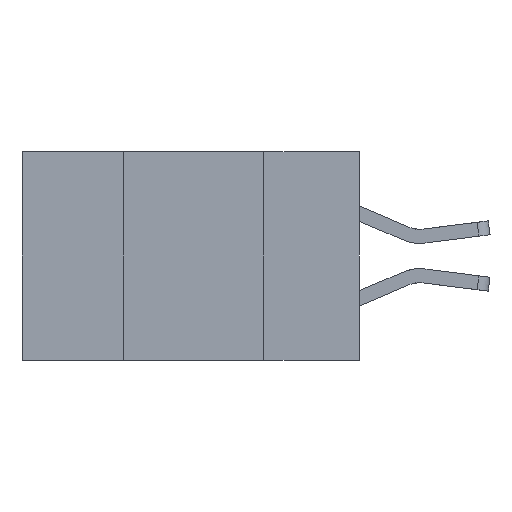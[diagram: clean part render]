
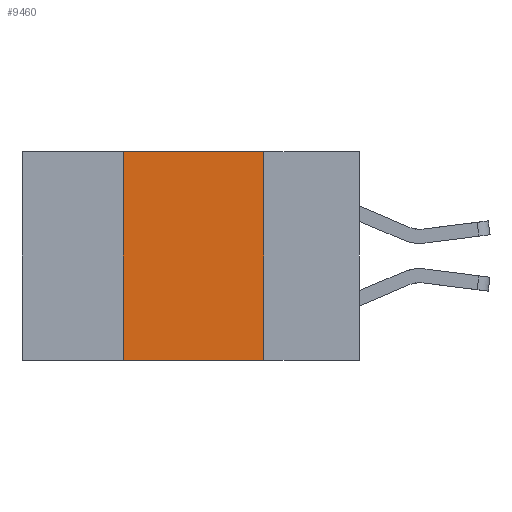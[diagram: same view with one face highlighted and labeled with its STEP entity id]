
A CAD part, left-side view. The second image highlights one B-rep face of the part: STEP entity #9460.
In plain terms, the highlighted planar face has unit normal (-1, 0, 0).
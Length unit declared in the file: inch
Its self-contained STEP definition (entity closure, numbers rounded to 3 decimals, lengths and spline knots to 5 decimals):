
#163 = EDGE_CURVE ( 'NONE', #6204, #4967, #328, .T. ) ;
#290 = CARTESIAN_POINT ( 'NONE',  ( 0., 0.6, 0. ) ) ;
#326 = ORIENTED_EDGE ( 'NONE', *, *, #1629, .F. ) ;
#328 = LINE ( 'NONE', #9199, #8879 ) ;
#525 = PLANE ( 'NONE',  #4400 ) ;
#876 = VECTOR ( 'NONE', #7766, 39.37008 ) ;
#1629 = EDGE_CURVE ( 'NONE', #8242, #8751, #9454, .T. ) ;
#1728 = DIRECTION ( 'NONE',  ( 0., 0., 1. ) ) ;
#2098 = ORIENTED_EDGE ( 'NONE', *, *, #6013, .F. ) ;
#2433 = CARTESIAN_POINT ( 'NONE',  ( 0., 0.17, -0.37 ) ) ;
#2679 = DIRECTION ( 'NONE',  ( 0., 0., -1. ) ) ;
#2828 = ORIENTED_EDGE ( 'NONE', *, *, #163, .F. ) ;
#3436 = EDGE_LOOP ( 'NONE', ( #326, #2098, #2828, #6363 ) ) ;
#4136 = DIRECTION ( 'NONE',  ( 0., -1., 0. ) ) ;
#4400 = AXIS2_PLACEMENT_3D ( 'NONE', #7452, #5819, #8094 ) ;
#4631 = CARTESIAN_POINT ( 'NONE',  ( 0., 0.42, 0. ) ) ;
#4692 = CARTESIAN_POINT ( 'NONE',  ( 0., 0.42, -0.37 ) ) ;
#4881 = LINE ( 'NONE', #9444, #8359 ) ;
#4967 = VERTEX_POINT ( 'NONE', #4631 ) ;
#5259 = VECTOR ( 'NONE', #2679, 39.37008 ) ;
#5319 = CARTESIAN_POINT ( 'NONE',  ( 0., 0.17, 0. ) ) ;
#5636 = LINE ( 'NONE', #290, #876 ) ;
#5819 = DIRECTION ( 'NONE',  ( 1., 0., 0. ) ) ;
#6013 = EDGE_CURVE ( 'NONE', #4967, #8242, #5636, .T. ) ;
#6204 = VERTEX_POINT ( 'NONE', #4692 ) ;
#6363 = ORIENTED_EDGE ( 'NONE', *, *, #9290, .T. ) ;
#7452 = CARTESIAN_POINT ( 'NONE',  ( 0., 0.6, 0. ) ) ;
#7766 = DIRECTION ( 'NONE',  ( 0., -1., 0. ) ) ;
#8094 = DIRECTION ( 'NONE',  ( 0., 0., -1. ) ) ;
#8166 = CARTESIAN_POINT ( 'NONE',  ( 0., 0.17, 0. ) ) ;
#8242 = VERTEX_POINT ( 'NONE', #5319 ) ;
#8359 = VECTOR ( 'NONE', #4136, 39.37008 ) ;
#8751 = VERTEX_POINT ( 'NONE', #2433 ) ;
#8879 = VECTOR ( 'NONE', #1728, 39.37008 ) ;
#9171 = FACE_OUTER_BOUND ( 'NONE', #3436, .T. ) ;
#9199 = CARTESIAN_POINT ( 'NONE',  ( 0., 0.42, 0. ) ) ;
#9290 = EDGE_CURVE ( 'NONE', #6204, #8751, #4881, .T. ) ;
#9444 = CARTESIAN_POINT ( 'NONE',  ( 0., 0.6, -0.37 ) ) ;
#9454 = LINE ( 'NONE', #8166, #5259 ) ;
#9460 = ADVANCED_FACE ( 'NONE', ( #9171 ), #525, .F. ) ;
